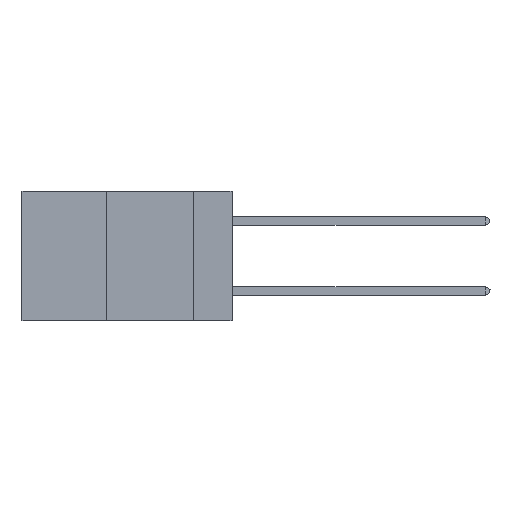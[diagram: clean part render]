
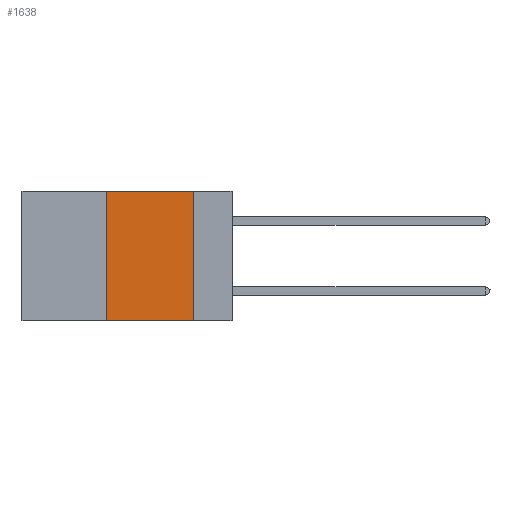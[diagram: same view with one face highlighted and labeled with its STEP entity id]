
A CAD part, left-side view. The second image highlights one B-rep face of the part: STEP entity #1638.
In plain terms, the highlighted planar face has unit normal (-1, 0, 0).
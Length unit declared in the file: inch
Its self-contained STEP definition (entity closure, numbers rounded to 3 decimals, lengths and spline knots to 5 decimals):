
#241 = CARTESIAN_POINT ( 'NONE',  ( 0., 0.11, -0.37 ) ) ;
#277 = CARTESIAN_POINT ( 'NONE',  ( 0., 0.36, 0. ) ) ;
#849 = VECTOR ( 'NONE', #6453, 39.37008 ) ;
#956 = DIRECTION ( 'NONE',  ( 0., 0., 1. ) ) ;
#992 = DIRECTION ( 'NONE',  ( 0., 0., -1. ) ) ;
#1069 = ORIENTED_EDGE ( 'NONE', *, *, #4645, .F. ) ;
#1089 = FACE_OUTER_BOUND ( 'NONE', #9893, .T. ) ;
#1539 = VERTEX_POINT ( 'NONE', #241 ) ;
#1638 = ADVANCED_FACE ( 'NONE', ( #1089 ), #6183, .F. ) ;
#1685 = LINE ( 'NONE', #10621, #4537 ) ;
#1697 = CARTESIAN_POINT ( 'NONE',  ( 0., 0.36, -0.37 ) ) ;
#2017 = EDGE_CURVE ( 'NONE', #3636, #1539, #7209, .T. ) ;
#2471 = CARTESIAN_POINT ( 'NONE',  ( 0., 0.36, 0. ) ) ;
#3636 = VERTEX_POINT ( 'NONE', #10424 ) ;
#4190 = AXIS2_PLACEMENT_3D ( 'NONE', #6977, #7032, #5268 ) ;
#4360 = ORIENTED_EDGE ( 'NONE', *, *, #2017, .F. ) ;
#4496 = DIRECTION ( 'NONE',  ( 0., -1., 0. ) ) ;
#4537 = VECTOR ( 'NONE', #4496, 39.37008 ) ;
#4645 = EDGE_CURVE ( 'NONE', #5424, #7599, #5460, .T. ) ;
#5268 = DIRECTION ( 'NONE',  ( 0., 0., -1. ) ) ;
#5364 = LINE ( 'NONE', #7987, #849 ) ;
#5424 = VERTEX_POINT ( 'NONE', #1697 ) ;
#5460 = LINE ( 'NONE', #277, #6748 ) ;
#5614 = CARTESIAN_POINT ( 'NONE',  ( 0., 0.11, 0. ) ) ;
#6183 = PLANE ( 'NONE',  #4190 ) ;
#6441 = EDGE_CURVE ( 'NONE', #7599, #3636, #5364, .T. ) ;
#6453 = DIRECTION ( 'NONE',  ( 0., -1., 0. ) ) ;
#6748 = VECTOR ( 'NONE', #956, 39.37008 ) ;
#6977 = CARTESIAN_POINT ( 'NONE',  ( 0., 0.6, 0. ) ) ;
#7032 = DIRECTION ( 'NONE',  ( 1., 0., 0. ) ) ;
#7209 = LINE ( 'NONE', #5614, #10901 ) ;
#7599 = VERTEX_POINT ( 'NONE', #2471 ) ;
#7987 = CARTESIAN_POINT ( 'NONE',  ( 0., 0.6, 0. ) ) ;
#8992 = ORIENTED_EDGE ( 'NONE', *, *, #6441, .F. ) ;
#9622 = ORIENTED_EDGE ( 'NONE', *, *, #10747, .T. ) ;
#9893 = EDGE_LOOP ( 'NONE', ( #4360, #8992, #1069, #9622 ) ) ;
#10424 = CARTESIAN_POINT ( 'NONE',  ( 0., 0.11, 0. ) ) ;
#10621 = CARTESIAN_POINT ( 'NONE',  ( 0., 0.6, -0.37 ) ) ;
#10747 = EDGE_CURVE ( 'NONE', #5424, #1539, #1685, .T. ) ;
#10901 = VECTOR ( 'NONE', #992, 39.37008 ) ;
